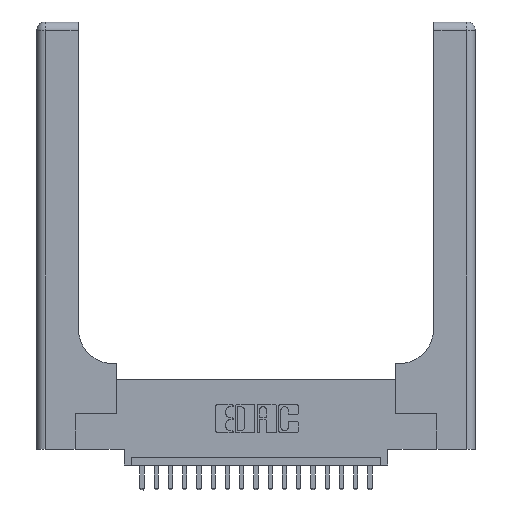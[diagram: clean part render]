
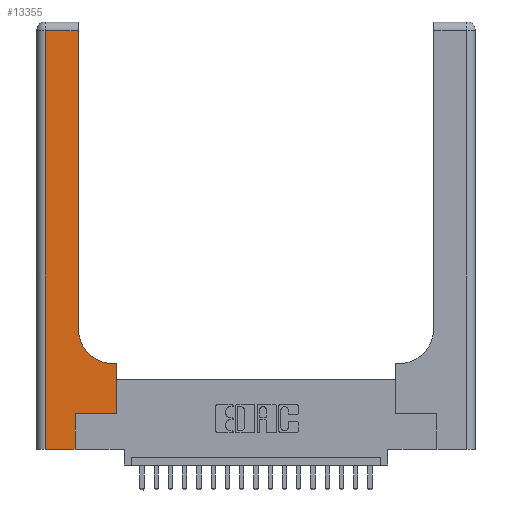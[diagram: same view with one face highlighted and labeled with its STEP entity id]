
A CAD part, top view. The second image highlights one B-rep face of the part: STEP entity #13355.
In plain terms, the highlighted planar face has unit normal (0, 0, 1).
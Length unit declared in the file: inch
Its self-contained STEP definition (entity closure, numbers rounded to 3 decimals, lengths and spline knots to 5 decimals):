
#326 = VERTEX_POINT ( 'NONE', #14741 ) ;
#377 = CIRCLE ( 'NONE', #8400, 0.25 ) ;
#926 = ORIENTED_EDGE ( 'NONE', *, *, #1035, .T. ) ;
#1035 = EDGE_CURVE ( 'NONE', #8885, #6199, #377, .T. ) ;
#1181 = DIRECTION ( 'NONE',  ( -1., 0., 0. ) ) ;
#1253 = DIRECTION ( 'NONE',  ( 0., 0., -1. ) ) ;
#1765 = EDGE_LOOP ( 'NONE', ( #13250, #5314, #21323, #18430, #16044, #21551, #10153, #9664, #926 ) ) ;
#2168 = VECTOR ( 'NONE', #7532, 39.37008 ) ;
#2231 = LINE ( 'NONE', #3948, #11796 ) ;
#2369 = DIRECTION ( 'NONE',  ( -1., 0., 0. ) ) ;
#2582 = VERTEX_POINT ( 'NONE', #4547 ) ;
#2636 = DIRECTION ( 'NONE',  ( 0., 1., 0. ) ) ;
#2727 = CARTESIAN_POINT ( 'NONE',  ( 0.06, 3., 0.37 ) ) ;
#2771 = CARTESIAN_POINT ( 'NONE',  ( 0.5585, 0.25, 0.37 ) ) ;
#2920 = EDGE_CURVE ( 'NONE', #326, #8885, #17109, .T. ) ;
#3100 = DIRECTION ( 'NONE',  ( 0., 0., -1. ) ) ;
#3159 = CARTESIAN_POINT ( 'NONE',  ( 0.269, 0., 0.37 ) ) ;
#3310 = VERTEX_POINT ( 'NONE', #8544 ) ;
#3627 = CARTESIAN_POINT ( 'NONE',  ( 0.269, 0.25, 0.37 ) ) ;
#3948 = CARTESIAN_POINT ( 'NONE',  ( 0., 2.94, 0.37 ) ) ;
#4299 = EDGE_CURVE ( 'NONE', #13952, #16173, #8213, .T. ) ;
#4429 = VECTOR ( 'NONE', #13646, 39.37008 ) ;
#4547 = CARTESIAN_POINT ( 'NONE',  ( 0.2915, 2.94, 0.37 ) ) ;
#4905 = EDGE_CURVE ( 'NONE', #5265, #3310, #10010, .T. ) ;
#5265 = VERTEX_POINT ( 'NONE', #11972 ) ;
#5314 = ORIENTED_EDGE ( 'NONE', *, *, #12796, .T. ) ;
#6137 = CARTESIAN_POINT ( 'NONE',  ( 0., 3., 0.37 ) ) ;
#6199 = VERTEX_POINT ( 'NONE', #17550 ) ;
#6636 = DIRECTION ( 'NONE',  ( 0., 1., 0. ) ) ;
#7053 = EDGE_CURVE ( 'NONE', #3310, #13952, #15382, .T. ) ;
#7532 = DIRECTION ( 'NONE',  ( 1., 0., 0. ) ) ;
#7617 = FACE_OUTER_BOUND ( 'NONE', #1765, .T. ) ;
#8057 = VECTOR ( 'NONE', #21580, 39.37008 ) ;
#8153 = EDGE_CURVE ( 'NONE', #16872, #326, #20888, .T. ) ;
#8213 = LINE ( 'NONE', #3159, #12903 ) ;
#8400 = AXIS2_PLACEMENT_3D ( 'NONE', #21169, #3100, #16361 ) ;
#8544 = CARTESIAN_POINT ( 'NONE',  ( 0.06, 0., 0.37 ) ) ;
#8885 = VERTEX_POINT ( 'NONE', #21099 ) ;
#9264 = EDGE_CURVE ( 'NONE', #16173, #16872, #20350, .T. ) ;
#9326 = VECTOR ( 'NONE', #20496, 39.37008 ) ;
#9664 = ORIENTED_EDGE ( 'NONE', *, *, #2920, .T. ) ;
#9846 = CARTESIAN_POINT ( 'NONE',  ( 0.2915, 3., 0.37 ) ) ;
#10010 = LINE ( 'NONE', #2727, #12857 ) ;
#10153 = ORIENTED_EDGE ( 'NONE', *, *, #8153, .T. ) ;
#11078 = PLANE ( 'NONE',  #14937 ) ;
#11796 = VECTOR ( 'NONE', #2369, 39.37008 ) ;
#11918 = VECTOR ( 'NONE', #2636, 39.37008 ) ;
#11972 = CARTESIAN_POINT ( 'NONE',  ( 0.06, 2.94, 0.37 ) ) ;
#12462 = LINE ( 'NONE', #9846, #8057 ) ;
#12677 = DIRECTION ( 'NONE',  ( 0., -1., 0. ) ) ;
#12699 = CARTESIAN_POINT ( 'NONE',  ( 0.5585, 0.25, 0.37 ) ) ;
#12796 = EDGE_CURVE ( 'NONE', #2582, #5265, #2231, .T. ) ;
#12857 = VECTOR ( 'NONE', #12677, 39.37008 ) ;
#12903 = VECTOR ( 'NONE', #6636, 39.37008 ) ;
#13250 = ORIENTED_EDGE ( 'NONE', *, *, #15901, .T. ) ;
#13355 = ADVANCED_FACE ( 'NONE', ( #7617 ), #11078, .F. ) ;
#13646 = DIRECTION ( 'NONE',  ( 1., 0., 0. ) ) ;
#13952 = VERTEX_POINT ( 'NONE', #15049 ) ;
#14014 = CARTESIAN_POINT ( 'NONE',  ( 0., 0., 0.37 ) ) ;
#14741 = CARTESIAN_POINT ( 'NONE',  ( 0.5585, 0.6, 0.37 ) ) ;
#14937 = AXIS2_PLACEMENT_3D ( 'NONE', #6137, #1253, #1181 ) ;
#15049 = CARTESIAN_POINT ( 'NONE',  ( 0.269, 0., 0.37 ) ) ;
#15382 = LINE ( 'NONE', #14014, #2168 ) ;
#15901 = EDGE_CURVE ( 'NONE', #6199, #2582, #12462, .T. ) ;
#16044 = ORIENTED_EDGE ( 'NONE', *, *, #4299, .T. ) ;
#16173 = VERTEX_POINT ( 'NONE', #3627 ) ;
#16361 = DIRECTION ( 'NONE',  ( 1., 0., 0. ) ) ;
#16872 = VERTEX_POINT ( 'NONE', #12699 ) ;
#17109 = LINE ( 'NONE', #18808, #9326 ) ;
#17550 = CARTESIAN_POINT ( 'NONE',  ( 0.2915, 0.85, 0.37 ) ) ;
#18430 = ORIENTED_EDGE ( 'NONE', *, *, #7053, .T. ) ;
#18661 = CARTESIAN_POINT ( 'NONE',  ( 0.269, 0.25, 0.37 ) ) ;
#18808 = CARTESIAN_POINT ( 'NONE',  ( 0.2915, 0.6, 0.37 ) ) ;
#20350 = LINE ( 'NONE', #18661, #4429 ) ;
#20496 = DIRECTION ( 'NONE',  ( -1., 0., 0. ) ) ;
#20888 = LINE ( 'NONE', #2771, #11918 ) ;
#21099 = CARTESIAN_POINT ( 'NONE',  ( 0.5415, 0.6, 0.37 ) ) ;
#21169 = CARTESIAN_POINT ( 'NONE',  ( 0.5415, 0.85, 0.37 ) ) ;
#21323 = ORIENTED_EDGE ( 'NONE', *, *, #4905, .T. ) ;
#21551 = ORIENTED_EDGE ( 'NONE', *, *, #9264, .T. ) ;
#21580 = DIRECTION ( 'NONE',  ( 0., 1., 0. ) ) ;
